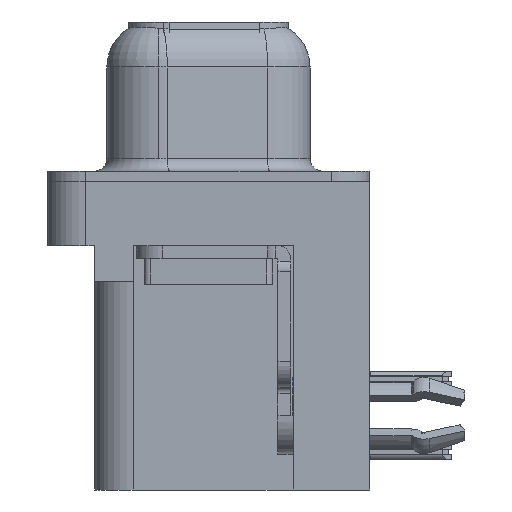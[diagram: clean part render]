
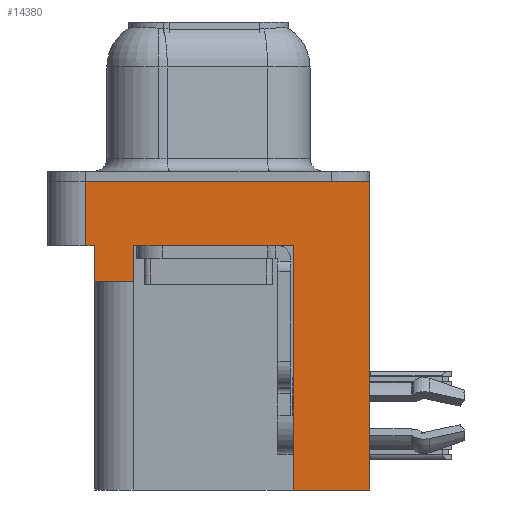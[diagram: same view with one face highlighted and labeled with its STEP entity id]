
A CAD part, left-side view. The second image highlights one B-rep face of the part: STEP entity #14380.
In plain terms, the highlighted planar face has unit normal (-1, 0, 0).
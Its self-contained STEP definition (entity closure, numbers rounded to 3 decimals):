
#76 = CARTESIAN_POINT ( 'NONE',  ( -3., 2.895, -3.9 ) ) ;
#561 = ORIENTED_EDGE ( 'NONE', *, *, #18897, .T. ) ;
#608 = LINE ( 'NONE', #17592, #6195 ) ;
#1083 = CARTESIAN_POINT ( 'NONE',  ( -3., -3.295, -12. ) ) ;
#1299 = DIRECTION ( 'NONE',  ( 0., -1., 0. ) ) ;
#1328 = DIRECTION ( 'NONE',  ( 0., 1., 0. ) ) ;
#1607 = VECTOR ( 'NONE', #2670, 1000. ) ;
#2594 = EDGE_CURVE ( 'NONE', #19484, #22935, #29732, .T. ) ;
#2670 = DIRECTION ( 'NONE',  ( 0., 0., 1. ) ) ;
#2723 = ORIENTED_EDGE ( 'NONE', *, *, #24125, .F. ) ;
#3362 = VECTOR ( 'NONE', #21099, 1000. ) ;
#3675 = CARTESIAN_POINT ( 'NONE',  ( -3., 4.775, -2.5 ) ) ;
#4868 = VECTOR ( 'NONE', #9408, 1000. ) ;
#5537 = DIRECTION ( 'NONE',  ( 0., 0., 1. ) ) ;
#5916 = EDGE_CURVE ( 'NONE', #25729, #23029, #7808, .T. ) ;
#6054 = CARTESIAN_POINT ( 'NONE',  ( -3., -3.295, -12. ) ) ;
#6076 = CARTESIAN_POINT ( 'NONE',  ( -3., -3.295, -2.5 ) ) ;
#6195 = VECTOR ( 'NONE', #1299, 1000. ) ;
#6459 = VERTEX_POINT ( 'NONE', #6076 ) ;
#6889 = LINE ( 'NONE', #23994, #22871 ) ;
#6891 = LINE ( 'NONE', #25216, #7264 ) ;
#6927 = CARTESIAN_POINT ( 'NONE',  ( -3., 4.425, -2.5 ) ) ;
#7264 = VECTOR ( 'NONE', #1328, 1000. ) ;
#7508 = ORIENTED_EDGE ( 'NONE', *, *, #17392, .F. ) ;
#7655 = ORIENTED_EDGE ( 'NONE', *, *, #12167, .F. ) ;
#7808 = LINE ( 'NONE', #29837, #15619 ) ;
#7965 = EDGE_CURVE ( 'NONE', #20680, #15455, #13435, .T. ) ;
#8782 = PLANE ( 'NONE',  #12308 ) ;
#8787 = LINE ( 'NONE', #8835, #11420 ) ;
#8835 = CARTESIAN_POINT ( 'NONE',  ( -3., -6.275, 0. ) ) ;
#8854 = DIRECTION ( 'NONE',  ( 0., -1., 0. ) ) ;
#8867 = LINE ( 'NONE', #15954, #3362 ) ;
#9408 = DIRECTION ( 'NONE',  ( 0., 0., 1. ) ) ;
#9704 = CARTESIAN_POINT ( 'NONE',  ( -3., 4.775, -2.5 ) ) ;
#10339 = VECTOR ( 'NONE', #5537, 1000. ) ;
#11377 = ORIENTED_EDGE ( 'NONE', *, *, #5916, .T. ) ;
#11420 = VECTOR ( 'NONE', #15973, 1000. ) ;
#11883 = VERTEX_POINT ( 'NONE', #6054 ) ;
#12167 = EDGE_CURVE ( 'NONE', #19484, #11883, #6891, .T. ) ;
#12308 = AXIS2_PLACEMENT_3D ( 'NONE', #16370, #30518, #16276 ) ;
#13435 = LINE ( 'NONE', #9704, #1607 ) ;
#13543 = EDGE_CURVE ( 'NONE', #20680, #24095, #27552, .T. ) ;
#13780 = CARTESIAN_POINT ( 'NONE',  ( -3., 2.895, -2.5 ) ) ;
#13850 = CARTESIAN_POINT ( 'NONE',  ( -3., -6.275, -2.5 ) ) ;
#14380 = ADVANCED_FACE ( 'NONE', ( #20534 ), #8782, .T. ) ;
#14464 = DIRECTION ( 'NONE',  ( 0., 1., 0. ) ) ;
#15455 = VERTEX_POINT ( 'NONE', #19924 ) ;
#15619 = VECTOR ( 'NONE', #22396, 1000. ) ;
#15664 = ORIENTED_EDGE ( 'NONE', *, *, #24818, .F. ) ;
#15954 = CARTESIAN_POINT ( 'NONE',  ( -3., 4.425, -3.9 ) ) ;
#15973 = DIRECTION ( 'NONE',  ( 0., -1., 0. ) ) ;
#16276 = DIRECTION ( 'NONE',  ( 0., 0., 1. ) ) ;
#16370 = CARTESIAN_POINT ( 'NONE',  ( -3., -6.275, -2.5 ) ) ;
#17392 = EDGE_CURVE ( 'NONE', #25729, #21633, #6889, .T. ) ;
#17497 = EDGE_LOOP ( 'NONE', ( #15664, #28360, #19588, #27960, #7508, #11377, #561, #2723, #7655, #30609 ) ) ;
#17592 = CARTESIAN_POINT ( 'NONE',  ( -3., -6.275, -2.5 ) ) ;
#18153 = LINE ( 'NONE', #1083, #10339 ) ;
#18790 = CARTESIAN_POINT ( 'NONE',  ( -3., -6.275, -2.5 ) ) ;
#18897 = EDGE_CURVE ( 'NONE', #23029, #6459, #608, .T. ) ;
#19484 = VERTEX_POINT ( 'NONE', #25595 ) ;
#19588 = ORIENTED_EDGE ( 'NONE', *, *, #13543, .T. ) ;
#19924 = CARTESIAN_POINT ( 'NONE',  ( -3., 4.775, 0. ) ) ;
#20501 = VECTOR ( 'NONE', #8854, 1000. ) ;
#20534 = FACE_OUTER_BOUND ( 'NONE', #17497, .T. ) ;
#20680 = VERTEX_POINT ( 'NONE', #3675 ) ;
#21099 = DIRECTION ( 'NONE',  ( 0., 0., 1. ) ) ;
#21633 = VERTEX_POINT ( 'NONE', #22853 ) ;
#22396 = DIRECTION ( 'NONE',  ( 0., 0., 1. ) ) ;
#22853 = CARTESIAN_POINT ( 'NONE',  ( -3., 4.425, -3.9 ) ) ;
#22871 = VECTOR ( 'NONE', #14464, 1000. ) ;
#22935 = VERTEX_POINT ( 'NONE', #28837 ) ;
#23029 = VERTEX_POINT ( 'NONE', #13780 ) ;
#23994 = CARTESIAN_POINT ( 'NONE',  ( -3., 4.425, -3.9 ) ) ;
#24095 = VERTEX_POINT ( 'NONE', #6927 ) ;
#24125 = EDGE_CURVE ( 'NONE', #11883, #6459, #18153, .T. ) ;
#24818 = EDGE_CURVE ( 'NONE', #15455, #22935, #8787, .T. ) ;
#25216 = CARTESIAN_POINT ( 'NONE',  ( -3., -3.295, -12. ) ) ;
#25595 = CARTESIAN_POINT ( 'NONE',  ( -3., -6.275, -12. ) ) ;
#25729 = VERTEX_POINT ( 'NONE', #76 ) ;
#27552 = LINE ( 'NONE', #13850, #20501 ) ;
#27960 = ORIENTED_EDGE ( 'NONE', *, *, #30316, .F. ) ;
#28360 = ORIENTED_EDGE ( 'NONE', *, *, #7965, .F. ) ;
#28837 = CARTESIAN_POINT ( 'NONE',  ( -3., -6.275, 0. ) ) ;
#29732 = LINE ( 'NONE', #18790, #4868 ) ;
#29837 = CARTESIAN_POINT ( 'NONE',  ( -3., 2.895, -3.9 ) ) ;
#30316 = EDGE_CURVE ( 'NONE', #21633, #24095, #8867, .T. ) ;
#30518 = DIRECTION ( 'NONE',  ( -1., 0., 0. ) ) ;
#30609 = ORIENTED_EDGE ( 'NONE', *, *, #2594, .T. ) ;
